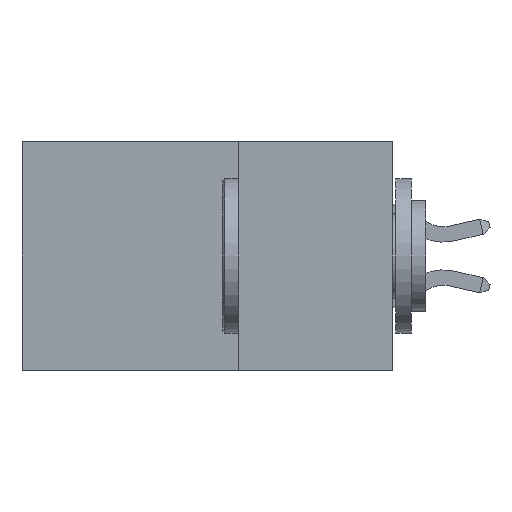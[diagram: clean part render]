
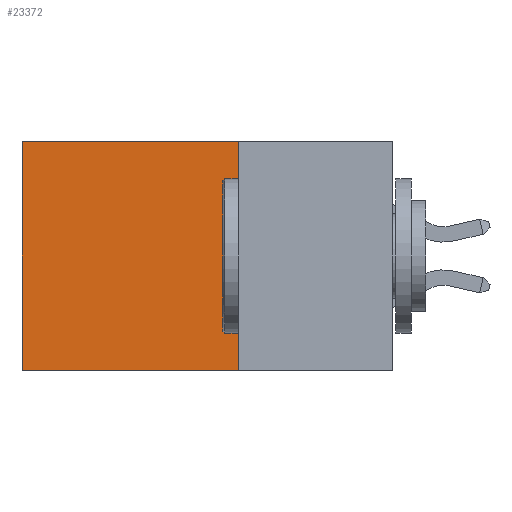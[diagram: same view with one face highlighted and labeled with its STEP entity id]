
A CAD part, left-side view. The second image highlights one B-rep face of the part: STEP entity #23372.
In plain terms, the highlighted planar face has unit normal (-1, 0, 0).
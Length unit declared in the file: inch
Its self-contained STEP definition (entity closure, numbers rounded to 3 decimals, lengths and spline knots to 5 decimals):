
#1196 = VERTEX_POINT ( 'NONE', #31082 ) ;
#1739 = DIRECTION ( 'NONE',  ( 0., 0., -1. ) ) ;
#4885 = DIRECTION ( 'NONE',  ( 0., 0., -1. ) ) ;
#6699 = CARTESIAN_POINT ( 'NONE',  ( 0.2875, 0.6, 0. ) ) ;
#6702 = VECTOR ( 'NONE', #16928, 39.37008 ) ;
#7566 = FACE_OUTER_BOUND ( 'NONE', #35573, .T. ) ;
#8780 = CARTESIAN_POINT ( 'NONE',  ( 0.2875, 0.25, -0.37 ) ) ;
#9317 = DIRECTION ( 'NONE',  ( 0., 1., 0. ) ) ;
#11253 = VECTOR ( 'NONE', #9317, 39.37008 ) ;
#14343 = CARTESIAN_POINT ( 'NONE',  ( 0.2875, 0.25, -0.37 ) ) ;
#14622 = VERTEX_POINT ( 'NONE', #6699 ) ;
#14638 = LINE ( 'NONE', #22751, #6702 ) ;
#14925 = LINE ( 'NONE', #8780, #22776 ) ;
#15757 = VERTEX_POINT ( 'NONE', #14343 ) ;
#16770 = PLANE ( 'NONE',  #24913 ) ;
#16928 = DIRECTION ( 'NONE',  ( 0., 0., -1. ) ) ;
#17337 = ORIENTED_EDGE ( 'NONE', *, *, #23703, .T. ) ;
#22707 = DIRECTION ( 'NONE',  ( 1., 0., 0. ) ) ;
#22716 = EDGE_CURVE ( 'NONE', #14622, #24065, #14638, .T. ) ;
#22751 = CARTESIAN_POINT ( 'NONE',  ( 0.2875, 0.6, 0. ) ) ;
#22776 = VECTOR ( 'NONE', #29502, 39.37008 ) ;
#23372 = ADVANCED_FACE ( 'NONE', ( #7566 ), #16770, .F. ) ;
#23703 = EDGE_CURVE ( 'NONE', #1196, #14622, #26085, .T. ) ;
#24065 = VERTEX_POINT ( 'NONE', #25490 ) ;
#24913 = AXIS2_PLACEMENT_3D ( 'NONE', #37231, #22707, #4885 ) ;
#25490 = CARTESIAN_POINT ( 'NONE',  ( 0.2875, 0.6, -0.37 ) ) ;
#25652 = EDGE_CURVE ( 'NONE', #15757, #24065, #14925, .T. ) ;
#26085 = LINE ( 'NONE', #27072, #11253 ) ;
#27072 = CARTESIAN_POINT ( 'NONE',  ( 0.2875, 0.25, 0. ) ) ;
#29502 = DIRECTION ( 'NONE',  ( 0., 1., 0. ) ) ;
#31082 = CARTESIAN_POINT ( 'NONE',  ( 0.2875, 0.25, 0. ) ) ;
#31534 = CARTESIAN_POINT ( 'NONE',  ( 0.2875, 0.25, 0. ) ) ;
#31909 = LINE ( 'NONE', #31534, #32853 ) ;
#32853 = VECTOR ( 'NONE', #1739, 39.37008 ) ;
#34142 = ORIENTED_EDGE ( 'NONE', *, *, #22716, .T. ) ;
#34715 = ORIENTED_EDGE ( 'NONE', *, *, #25652, .F. ) ;
#35573 = EDGE_LOOP ( 'NONE', ( #34142, #34715, #38257, #17337 ) ) ;
#35810 = EDGE_CURVE ( 'NONE', #1196, #15757, #31909, .T. ) ;
#37231 = CARTESIAN_POINT ( 'NONE',  ( 0.2875, 0.25, 0. ) ) ;
#38257 = ORIENTED_EDGE ( 'NONE', *, *, #35810, .F. ) ;
